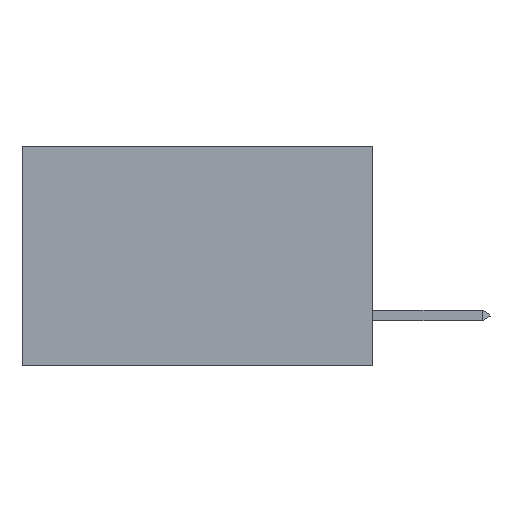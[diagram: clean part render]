
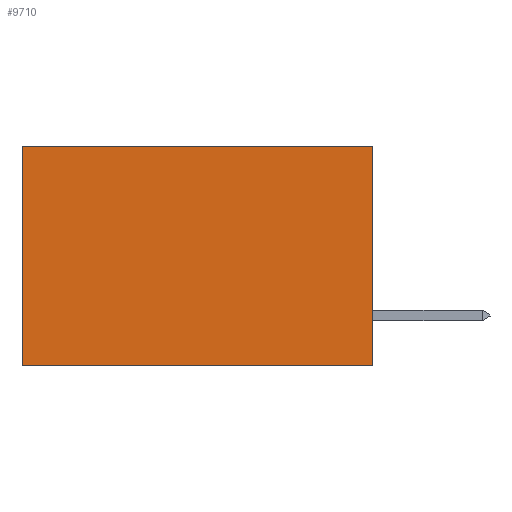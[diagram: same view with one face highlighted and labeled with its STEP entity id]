
A CAD part, left-side view. The second image highlights one B-rep face of the part: STEP entity #9710.
In plain terms, the highlighted planar face has unit normal (-1, 0, 0).
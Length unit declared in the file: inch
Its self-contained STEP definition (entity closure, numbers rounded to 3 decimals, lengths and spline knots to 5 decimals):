
#283 = CARTESIAN_POINT ( 'NONE',  ( 0.277, 0., -0.37 ) ) ;
#578 = EDGE_CURVE ( 'NONE', #10201, #896, #3028, .T. ) ;
#896 = VERTEX_POINT ( 'NONE', #8246 ) ;
#1584 = VECTOR ( 'NONE', #5014, 39.37008 ) ;
#1929 = ORIENTED_EDGE ( 'NONE', *, *, #12160, .F. ) ;
#2179 = EDGE_CURVE ( 'NONE', #10201, #4700, #11167, .T. ) ;
#2256 = CARTESIAN_POINT ( 'NONE',  ( 0.277, 0., -0.37 ) ) ;
#2393 = DIRECTION ( 'NONE',  ( 1., 0., 0. ) ) ;
#2403 = DIRECTION ( 'NONE',  ( 0., 1., 0. ) ) ;
#2531 = DIRECTION ( 'NONE',  ( 0., 0., -1. ) ) ;
#2563 = CARTESIAN_POINT ( 'NONE',  ( 0.277, 0., 0. ) ) ;
#3028 = LINE ( 'NONE', #2256, #10373 ) ;
#3168 = VERTEX_POINT ( 'NONE', #6893 ) ;
#4419 = ORIENTED_EDGE ( 'NONE', *, *, #578, .F. ) ;
#4700 = VERTEX_POINT ( 'NONE', #6371 ) ;
#5014 = DIRECTION ( 'NONE',  ( 0., 1., 0. ) ) ;
#6136 = AXIS2_PLACEMENT_3D ( 'NONE', #8086, #2393, #9059 ) ;
#6140 = PLANE ( 'NONE',  #6136 ) ;
#6329 = FACE_OUTER_BOUND ( 'NONE', #8174, .T. ) ;
#6371 = CARTESIAN_POINT ( 'NONE',  ( 0.277, 0.59, 0. ) ) ;
#6453 = EDGE_CURVE ( 'NONE', #4700, #3168, #7772, .T. ) ;
#6893 = CARTESIAN_POINT ( 'NONE',  ( 0.277, 0.59, -0.37 ) ) ;
#7173 = VECTOR ( 'NONE', #10414, 39.37008 ) ;
#7772 = LINE ( 'NONE', #10316, #7173 ) ;
#8086 = CARTESIAN_POINT ( 'NONE',  ( 0.277, 0., -0.37 ) ) ;
#8174 = EDGE_LOOP ( 'NONE', ( #8955, #1929, #4419, #11967 ) ) ;
#8246 = CARTESIAN_POINT ( 'NONE',  ( 0.277, 0., -0.37 ) ) ;
#8664 = VECTOR ( 'NONE', #2403, 39.37008 ) ;
#8955 = ORIENTED_EDGE ( 'NONE', *, *, #6453, .T. ) ;
#9059 = DIRECTION ( 'NONE',  ( 0., 0., -1. ) ) ;
#9710 = ADVANCED_FACE ( 'NONE', ( #6329 ), #6140, .F. ) ;
#10201 = VERTEX_POINT ( 'NONE', #10721 ) ;
#10316 = CARTESIAN_POINT ( 'NONE',  ( 0.277, 0.59, -0.37 ) ) ;
#10373 = VECTOR ( 'NONE', #2531, 39.37008 ) ;
#10414 = DIRECTION ( 'NONE',  ( 0., 0., -1. ) ) ;
#10721 = CARTESIAN_POINT ( 'NONE',  ( 0.277, 0., 0. ) ) ;
#11167 = LINE ( 'NONE', #2563, #8664 ) ;
#11762 = LINE ( 'NONE', #283, #1584 ) ;
#11967 = ORIENTED_EDGE ( 'NONE', *, *, #2179, .T. ) ;
#12160 = EDGE_CURVE ( 'NONE', #896, #3168, #11762, .T. ) ;
